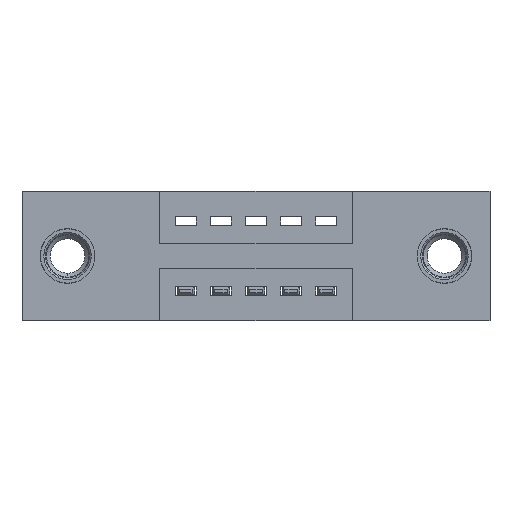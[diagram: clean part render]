
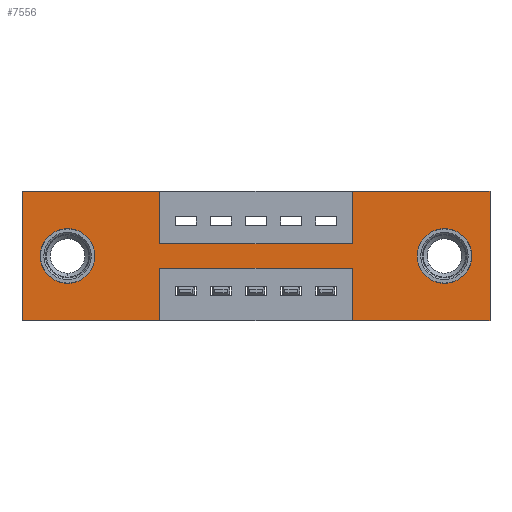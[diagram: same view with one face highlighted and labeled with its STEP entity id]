
A CAD part, front view. The second image highlights one B-rep face of the part: STEP entity #7556.
In plain terms, the highlighted planar face has unit normal (0, -1, 0).
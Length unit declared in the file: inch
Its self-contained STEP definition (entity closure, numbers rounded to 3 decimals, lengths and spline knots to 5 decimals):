
#79 = CARTESIAN_POINT ( 'NONE',  ( 0.3925, 0., -0.22 ) ) ;
#80 = DIRECTION ( 'NONE',  ( 1., 0., 0. ) ) ;
#221 = VERTEX_POINT ( 'NONE', #7722 ) ;
#501 = LINE ( 'NONE', #4760, #7817 ) ;
#512 = ORIENTED_EDGE ( 'NONE', *, *, #4108, .T. ) ;
#718 = EDGE_CURVE ( 'NONE', #9496, #5478, #6460, .T. ) ;
#807 = VERTEX_POINT ( 'NONE', #7286 ) ;
#897 = VERTEX_POINT ( 'NONE', #4083 ) ;
#951 = DIRECTION ( 'NONE',  ( 1., 0., 0. ) ) ;
#1029 = EDGE_CURVE ( 'NONE', #2018, #3954, #4723, .T. ) ;
#1055 = CARTESIAN_POINT ( 'NONE',  ( 1.205, 0., -0.263 ) ) ;
#1077 = CARTESIAN_POINT ( 'NONE',  ( 0.13, 0., -0.185 ) ) ;
#1124 = DIRECTION ( 'NONE',  ( 0., -1., 0. ) ) ;
#1241 = CARTESIAN_POINT ( 'NONE',  ( 1.335, 0., 0. ) ) ;
#1304 = ORIENTED_EDGE ( 'NONE', *, *, #6028, .F. ) ;
#1356 = EDGE_LOOP ( 'NONE', ( #5808, #6069, #1304, #6573, #5403, #8204, #8800, #6140, #1642, #6215, #6303, #5523 ) ) ;
#1436 = CARTESIAN_POINT ( 'NONE',  ( 0.3925, 0., 0. ) ) ;
#1437 = VECTOR ( 'NONE', #4273, 39.37008 ) ;
#1471 = EDGE_CURVE ( 'NONE', #3954, #9496, #6561, .T. ) ;
#1508 = VECTOR ( 'NONE', #5586, 39.37008 ) ;
#1521 = DIRECTION ( 'NONE',  ( -1., 0., 0. ) ) ;
#1628 = CARTESIAN_POINT ( 'NONE',  ( 0., 0., 0. ) ) ;
#1642 = ORIENTED_EDGE ( 'NONE', *, *, #718, .F. ) ;
#1776 = CARTESIAN_POINT ( 'NONE',  ( 0.3925, 0., -0.15 ) ) ;
#1788 = CARTESIAN_POINT ( 'NONE',  ( 0.9425, 0., -0.22 ) ) ;
#1831 = CIRCLE ( 'NONE', #4956, 0.078 ) ;
#1854 = CARTESIAN_POINT ( 'NONE',  ( 0.9425, 0., -0.37 ) ) ;
#1890 = VECTOR ( 'NONE', #80, 39.37008 ) ;
#1901 = VERTEX_POINT ( 'NONE', #1788 ) ;
#2018 = VERTEX_POINT ( 'NONE', #2472 ) ;
#2030 = VECTOR ( 'NONE', #6662, 39.37008 ) ;
#2068 = CARTESIAN_POINT ( 'NONE',  ( 0.13, 0., -0.185 ) ) ;
#2134 = VECTOR ( 'NONE', #5557, 39.37008 ) ;
#2152 = LINE ( 'NONE', #1241, #1437 ) ;
#2429 = EDGE_LOOP ( 'NONE', ( #512, #6554 ) ) ;
#2472 = CARTESIAN_POINT ( 'NONE',  ( 0., 0., -0.37 ) ) ;
#2475 = VECTOR ( 'NONE', #2739, 39.37008 ) ;
#2502 = DIRECTION ( 'NONE',  ( 0., 1., 0. ) ) ;
#2572 = EDGE_CURVE ( 'NONE', #6291, #8696, #6557, .T. ) ;
#2739 = DIRECTION ( 'NONE',  ( -1., 0., 0. ) ) ;
#2975 = CARTESIAN_POINT ( 'NONE',  ( 0.9425, 0., -0.37 ) ) ;
#3053 = LINE ( 'NONE', #6361, #2475 ) ;
#3369 = ORIENTED_EDGE ( 'NONE', *, *, #8685, .T. ) ;
#3538 = DIRECTION ( 'NONE',  ( 0., 1., 0. ) ) ;
#3638 = CIRCLE ( 'NONE', #6314, 0.078 ) ;
#3735 = VECTOR ( 'NONE', #7572, 39.37008 ) ;
#3804 = VECTOR ( 'NONE', #5450, 39.37008 ) ;
#3807 = LINE ( 'NONE', #1776, #5427 ) ;
#3954 = VERTEX_POINT ( 'NONE', #4479 ) ;
#3969 = VECTOR ( 'NONE', #1521, 39.37008 ) ;
#4022 = FACE_BOUND ( 'NONE', #8374, .T. ) ;
#4050 = DIRECTION ( 'NONE',  ( 0., 1., 0. ) ) ;
#4083 = CARTESIAN_POINT ( 'NONE',  ( 0.9425, 0., -0.15 ) ) ;
#4090 = CARTESIAN_POINT ( 'NONE',  ( 0., 0., -0.37 ) ) ;
#4108 = EDGE_CURVE ( 'NONE', #4144, #7167, #3638, .T. ) ;
#4131 = FACE_BOUND ( 'NONE', #2429, .T. ) ;
#4144 = VERTEX_POINT ( 'NONE', #7079 ) ;
#4273 = DIRECTION ( 'NONE',  ( 0., 0., -1. ) ) ;
#4287 = EDGE_CURVE ( 'NONE', #4482, #2018, #3053, .T. ) ;
#4313 = LINE ( 'NONE', #79, #3969 ) ;
#4479 = CARTESIAN_POINT ( 'NONE',  ( 0., 0., 0. ) ) ;
#4482 = VERTEX_POINT ( 'NONE', #7396 ) ;
#4511 = VECTOR ( 'NONE', #5500, 39.37008 ) ;
#4675 = EDGE_CURVE ( 'NONE', #1901, #221, #4313, .T. ) ;
#4723 = LINE ( 'NONE', #1628, #3804 ) ;
#4760 = CARTESIAN_POINT ( 'NONE',  ( 0.9425, 0., 0. ) ) ;
#4783 = EDGE_CURVE ( 'NONE', #807, #9369, #5600, .T. ) ;
#4815 = CARTESIAN_POINT ( 'NONE',  ( 1.205, 0., -0.185 ) ) ;
#4832 = DIRECTION ( 'NONE',  ( 0., 0., 1. ) ) ;
#4940 = CARTESIAN_POINT ( 'NONE',  ( 0.13, 0., -0.107 ) ) ;
#4956 = AXIS2_PLACEMENT_3D ( 'NONE', #9551, #3538, #5726 ) ;
#4967 = CARTESIAN_POINT ( 'NONE',  ( 0.3925, 0., 0. ) ) ;
#5009 = CARTESIAN_POINT ( 'NONE',  ( 0.13, 0., -0.263 ) ) ;
#5403 = ORIENTED_EDGE ( 'NONE', *, *, #8377, .F. ) ;
#5427 = VECTOR ( 'NONE', #951, 39.37008 ) ;
#5450 = DIRECTION ( 'NONE',  ( 0., 0., 1. ) ) ;
#5478 = VERTEX_POINT ( 'NONE', #7665 ) ;
#5500 = DIRECTION ( 'NONE',  ( 0., 0., -1. ) ) ;
#5523 = ORIENTED_EDGE ( 'NONE', *, *, #4287, .F. ) ;
#5524 = CARTESIAN_POINT ( 'NONE',  ( 0., 0., 0. ) ) ;
#5552 = DIRECTION ( 'NONE',  ( 0., 0., -1. ) ) ;
#5557 = DIRECTION ( 'NONE',  ( 1., 0., 0. ) ) ;
#5586 = DIRECTION ( 'NONE',  ( -1., 0., 0. ) ) ;
#5600 = LINE ( 'NONE', #4090, #1508 ) ;
#5726 = DIRECTION ( 'NONE',  ( 0., 0., -1. ) ) ;
#5808 = ORIENTED_EDGE ( 'NONE', *, *, #6812, .F. ) ;
#5870 = DIRECTION ( 'NONE',  ( 0., 1., 0. ) ) ;
#5902 = LINE ( 'NONE', #2975, #3735 ) ;
#5962 = AXIS2_PLACEMENT_3D ( 'NONE', #1077, #4050, #6979 ) ;
#6028 = EDGE_CURVE ( 'NONE', #9369, #1901, #5902, .T. ) ;
#6069 = ORIENTED_EDGE ( 'NONE', *, *, #4675, .F. ) ;
#6140 = ORIENTED_EDGE ( 'NONE', *, *, #8134, .F. ) ;
#6215 = ORIENTED_EDGE ( 'NONE', *, *, #1471, .F. ) ;
#6231 = DIRECTION ( 'NONE',  ( 0., 0., -1. ) ) ;
#6236 = EDGE_CURVE ( 'NONE', #7167, #4144, #1831, .T. ) ;
#6267 = CARTESIAN_POINT ( 'NONE',  ( 1.335, 0., 0. ) ) ;
#6291 = VERTEX_POINT ( 'NONE', #7466 ) ;
#6303 = ORIENTED_EDGE ( 'NONE', *, *, #1029, .F. ) ;
#6314 = AXIS2_PLACEMENT_3D ( 'NONE', #4815, #2502, #6231 ) ;
#6331 = VERTEX_POINT ( 'NONE', #5009 ) ;
#6361 = CARTESIAN_POINT ( 'NONE',  ( 0., 0., -0.37 ) ) ;
#6460 = LINE ( 'NONE', #1436, #2030 ) ;
#6554 = ORIENTED_EDGE ( 'NONE', *, *, #6236, .T. ) ;
#6557 = LINE ( 'NONE', #6832, #1890 ) ;
#6561 = LINE ( 'NONE', #5524, #2134 ) ;
#6564 = AXIS2_PLACEMENT_3D ( 'NONE', #2068, #5870, #6636 ) ;
#6573 = ORIENTED_EDGE ( 'NONE', *, *, #4783, .F. ) ;
#6636 = DIRECTION ( 'NONE',  ( 0., 0., 1. ) ) ;
#6640 = AXIS2_PLACEMENT_3D ( 'NONE', #7003, #1124, #5552 ) ;
#6662 = DIRECTION ( 'NONE',  ( 0., 0., -1. ) ) ;
#6812 = EDGE_CURVE ( 'NONE', #221, #4482, #8546, .T. ) ;
#6832 = CARTESIAN_POINT ( 'NONE',  ( 0., 0., 0. ) ) ;
#6968 = CARTESIAN_POINT ( 'NONE',  ( 0.3925, 0., -0.37 ) ) ;
#6979 = DIRECTION ( 'NONE',  ( 0., 0., 1. ) ) ;
#7003 = CARTESIAN_POINT ( 'NONE',  ( 0., 0., -0.37 ) ) ;
#7079 = CARTESIAN_POINT ( 'NONE',  ( 1.205, 0., -0.107 ) ) ;
#7167 = VERTEX_POINT ( 'NONE', #1055 ) ;
#7197 = EDGE_CURVE ( 'NONE', #897, #6291, #501, .T. ) ;
#7286 = CARTESIAN_POINT ( 'NONE',  ( 1.335, 0., -0.37 ) ) ;
#7395 = EDGE_CURVE ( 'NONE', #6331, #7741, #9233, .T. ) ;
#7396 = CARTESIAN_POINT ( 'NONE',  ( 0.3925, 0., -0.37 ) ) ;
#7466 = CARTESIAN_POINT ( 'NONE',  ( 0.9425, 0., 0. ) ) ;
#7556 = ADVANCED_FACE ( 'NONE', ( #4131, #4022, #9580 ), #9435, .T. ) ;
#7572 = DIRECTION ( 'NONE',  ( 0., 0., 1. ) ) ;
#7665 = CARTESIAN_POINT ( 'NONE',  ( 0.3925, 0., -0.15 ) ) ;
#7722 = CARTESIAN_POINT ( 'NONE',  ( 0.3925, 0., -0.22 ) ) ;
#7741 = VERTEX_POINT ( 'NONE', #4940 ) ;
#7817 = VECTOR ( 'NONE', #4832, 39.37008 ) ;
#8066 = CIRCLE ( 'NONE', #5962, 0.078 ) ;
#8134 = EDGE_CURVE ( 'NONE', #5478, #897, #3807, .T. ) ;
#8204 = ORIENTED_EDGE ( 'NONE', *, *, #2572, .F. ) ;
#8374 = EDGE_LOOP ( 'NONE', ( #3369, #9423 ) ) ;
#8377 = EDGE_CURVE ( 'NONE', #8696, #807, #2152, .T. ) ;
#8546 = LINE ( 'NONE', #6968, #4511 ) ;
#8685 = EDGE_CURVE ( 'NONE', #7741, #6331, #8066, .T. ) ;
#8696 = VERTEX_POINT ( 'NONE', #6267 ) ;
#8800 = ORIENTED_EDGE ( 'NONE', *, *, #7197, .F. ) ;
#9233 = CIRCLE ( 'NONE', #6564, 0.078 ) ;
#9369 = VERTEX_POINT ( 'NONE', #1854 ) ;
#9423 = ORIENTED_EDGE ( 'NONE', *, *, #7395, .T. ) ;
#9435 = PLANE ( 'NONE',  #6640 ) ;
#9496 = VERTEX_POINT ( 'NONE', #4967 ) ;
#9551 = CARTESIAN_POINT ( 'NONE',  ( 1.205, 0., -0.185 ) ) ;
#9580 = FACE_OUTER_BOUND ( 'NONE', #1356, .T. ) ;
